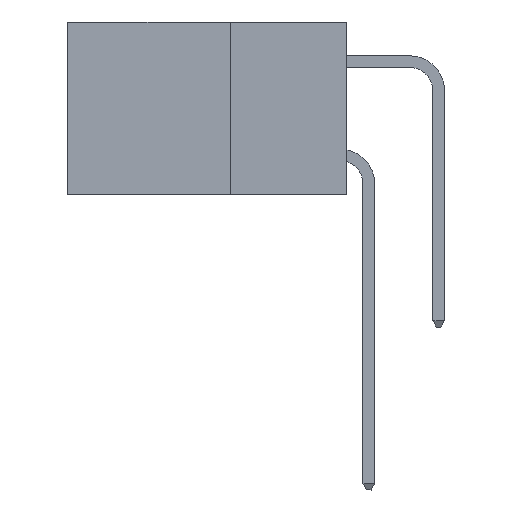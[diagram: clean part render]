
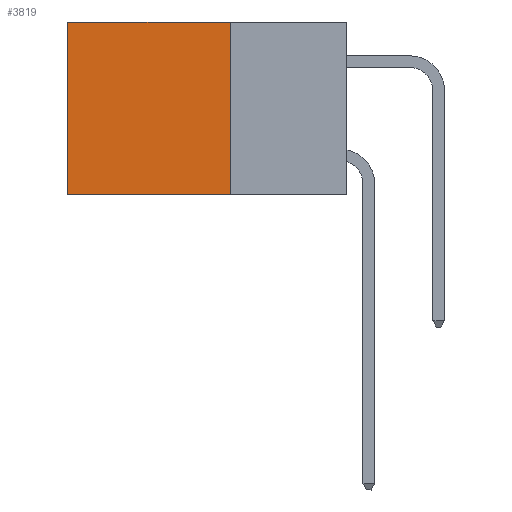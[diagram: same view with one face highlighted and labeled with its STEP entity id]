
A CAD part, left-side view. The second image highlights one B-rep face of the part: STEP entity #3819.
In plain terms, the highlighted planar face has unit normal (-1, 0, 0).
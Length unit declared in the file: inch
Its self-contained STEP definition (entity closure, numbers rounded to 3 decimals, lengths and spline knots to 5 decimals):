
#523 = DIRECTION ( 'NONE',  ( 0., 0., -1. ) ) ;
#608 = VECTOR ( 'NONE', #2057, 39.37008 ) ;
#690 = VERTEX_POINT ( 'NONE', #17259 ) ;
#731 = CARTESIAN_POINT ( 'NONE',  ( 0.2875, 0.6, 0. ) ) ;
#1300 = ORIENTED_EDGE ( 'NONE', *, *, #18656, .T. ) ;
#2057 = DIRECTION ( 'NONE',  ( 0., 1., 0. ) ) ;
#2136 = CARTESIAN_POINT ( 'NONE',  ( 0.2875, 0.25, 0. ) ) ;
#3819 = ADVANCED_FACE ( 'NONE', ( #20230 ), #5847, .F. ) ;
#4054 = VECTOR ( 'NONE', #5164, 39.37008 ) ;
#4631 = CARTESIAN_POINT ( 'NONE',  ( 0.2875, 0.25, -0.37 ) ) ;
#4856 = AXIS2_PLACEMENT_3D ( 'NONE', #7205, #8894, #16882 ) ;
#5164 = DIRECTION ( 'NONE',  ( 0., 1., 0. ) ) ;
#5847 = PLANE ( 'NONE',  #4856 ) ;
#6116 = CARTESIAN_POINT ( 'NONE',  ( 0.2875, 0.6, -0.37 ) ) ;
#6708 = VECTOR ( 'NONE', #18101, 39.37008 ) ;
#7205 = CARTESIAN_POINT ( 'NONE',  ( 0.2875, 0.25, 0. ) ) ;
#7703 = ORIENTED_EDGE ( 'NONE', *, *, #13559, .F. ) ;
#8894 = DIRECTION ( 'NONE',  ( 1., 0., 0. ) ) ;
#9517 = VERTEX_POINT ( 'NONE', #18166 ) ;
#9819 = LINE ( 'NONE', #2136, #6708 ) ;
#9976 = EDGE_CURVE ( 'NONE', #9517, #690, #16664, .T. ) ;
#10086 = LINE ( 'NONE', #731, #19567 ) ;
#10733 = ORIENTED_EDGE ( 'NONE', *, *, #14470, .F. ) ;
#13559 = EDGE_CURVE ( 'NONE', #9517, #16395, #9819, .T. ) ;
#13640 = EDGE_LOOP ( 'NONE', ( #1300, #10733, #7703, #20518 ) ) ;
#14470 = EDGE_CURVE ( 'NONE', #16395, #20207, #16830, .T. ) ;
#16395 = VERTEX_POINT ( 'NONE', #4631 ) ;
#16457 = CARTESIAN_POINT ( 'NONE',  ( 0.2875, 0.25, 0. ) ) ;
#16664 = LINE ( 'NONE', #16457, #608 ) ;
#16830 = LINE ( 'NONE', #19661, #4054 ) ;
#16882 = DIRECTION ( 'NONE',  ( 0., 0., -1. ) ) ;
#17259 = CARTESIAN_POINT ( 'NONE',  ( 0.2875, 0.6, 0. ) ) ;
#18101 = DIRECTION ( 'NONE',  ( 0., 0., -1. ) ) ;
#18166 = CARTESIAN_POINT ( 'NONE',  ( 0.2875, 0.25, 0. ) ) ;
#18656 = EDGE_CURVE ( 'NONE', #690, #20207, #10086, .T. ) ;
#19567 = VECTOR ( 'NONE', #523, 39.37008 ) ;
#19661 = CARTESIAN_POINT ( 'NONE',  ( 0.2875, 0.25, -0.37 ) ) ;
#20207 = VERTEX_POINT ( 'NONE', #6116 ) ;
#20230 = FACE_OUTER_BOUND ( 'NONE', #13640, .T. ) ;
#20518 = ORIENTED_EDGE ( 'NONE', *, *, #9976, .T. ) ;
